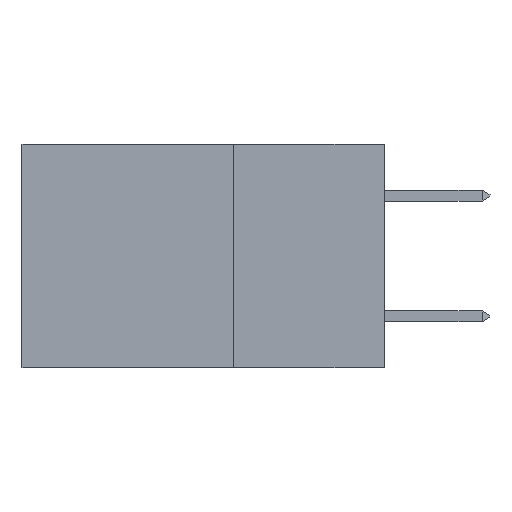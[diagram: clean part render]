
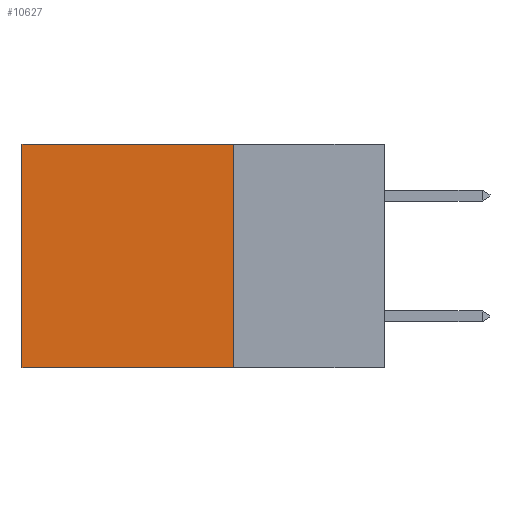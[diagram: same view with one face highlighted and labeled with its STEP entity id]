
A CAD part, left-side view. The second image highlights one B-rep face of the part: STEP entity #10627.
In plain terms, the highlighted planar face has unit normal (-1, 0, 0).
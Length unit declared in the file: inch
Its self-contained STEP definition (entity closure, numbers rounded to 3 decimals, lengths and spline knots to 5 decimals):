
#14 = CARTESIAN_POINT ( 'NONE',  ( 0.2875, 0.6, 0. ) ) ;
#620 = VECTOR ( 'NONE', #7017, 39.37008 ) ;
#1010 = DIRECTION ( 'NONE',  ( 0., 0., -1. ) ) ;
#1023 = PLANE ( 'NONE',  #3421 ) ;
#1038 = DIRECTION ( 'NONE',  ( 1., 0., 0. ) ) ;
#1330 = EDGE_CURVE ( 'NONE', #5789, #3937, #11184, .T. ) ;
#1540 = ORIENTED_EDGE ( 'NONE', *, *, #1330, .F. ) ;
#1653 = CARTESIAN_POINT ( 'NONE',  ( 0.2875, 0.25, 0. ) ) ;
#1745 = CARTESIAN_POINT ( 'NONE',  ( 0.2875, 0.25, 0. ) ) ;
#1829 = VERTEX_POINT ( 'NONE', #11819 ) ;
#2525 = CARTESIAN_POINT ( 'NONE',  ( 0.2875, 0.6, -0.37 ) ) ;
#2667 = CARTESIAN_POINT ( 'NONE',  ( 0.2875, 0.6, 0. ) ) ;
#3421 = AXIS2_PLACEMENT_3D ( 'NONE', #1653, #1038, #1010 ) ;
#3803 = DIRECTION ( 'NONE',  ( 0., 0., -1. ) ) ;
#3937 = VERTEX_POINT ( 'NONE', #2525 ) ;
#3947 = VECTOR ( 'NONE', #6909, 39.37008 ) ;
#4145 = FACE_OUTER_BOUND ( 'NONE', #5250, .T. ) ;
#4586 = LINE ( 'NONE', #1745, #7086 ) ;
#4881 = VECTOR ( 'NONE', #3803, 39.37008 ) ;
#4994 = EDGE_CURVE ( 'NONE', #1829, #5789, #7907, .T. ) ;
#5034 = EDGE_CURVE ( 'NONE', #1829, #9708, #4586, .T. ) ;
#5191 = CARTESIAN_POINT ( 'NONE',  ( 0.2875, 0.25, -0.37 ) ) ;
#5250 = EDGE_LOOP ( 'NONE', ( #11412, #1540, #6526, #5257 ) ) ;
#5257 = ORIENTED_EDGE ( 'NONE', *, *, #5034, .T. ) ;
#5349 = EDGE_CURVE ( 'NONE', #9708, #3937, #8444, .T. ) ;
#5789 = VERTEX_POINT ( 'NONE', #5191 ) ;
#5993 = DIRECTION ( 'NONE',  ( 0., 1., 0. ) ) ;
#6526 = ORIENTED_EDGE ( 'NONE', *, *, #4994, .F. ) ;
#6909 = DIRECTION ( 'NONE',  ( 0., 1., 0. ) ) ;
#7017 = DIRECTION ( 'NONE',  ( 0., 0., -1. ) ) ;
#7086 = VECTOR ( 'NONE', #5993, 39.37008 ) ;
#7907 = LINE ( 'NONE', #10420, #4881 ) ;
#8444 = LINE ( 'NONE', #14, #620 ) ;
#9708 = VERTEX_POINT ( 'NONE', #2667 ) ;
#10420 = CARTESIAN_POINT ( 'NONE',  ( 0.2875, 0.25, 0. ) ) ;
#10627 = ADVANCED_FACE ( 'NONE', ( #4145 ), #1023, .F. ) ;
#10867 = CARTESIAN_POINT ( 'NONE',  ( 0.2875, 0.25, -0.37 ) ) ;
#11184 = LINE ( 'NONE', #10867, #3947 ) ;
#11412 = ORIENTED_EDGE ( 'NONE', *, *, #5349, .T. ) ;
#11819 = CARTESIAN_POINT ( 'NONE',  ( 0.2875, 0.25, 0. ) ) ;
